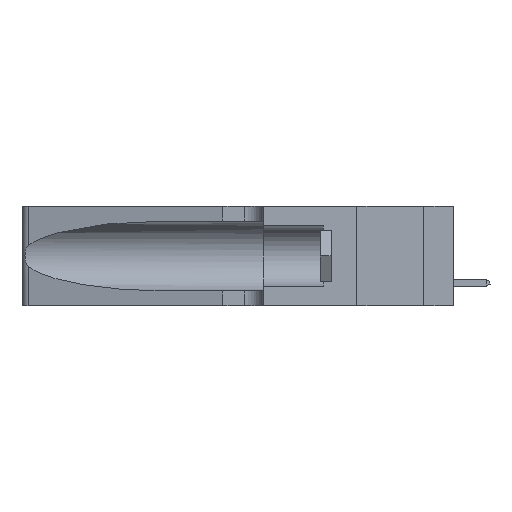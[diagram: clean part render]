
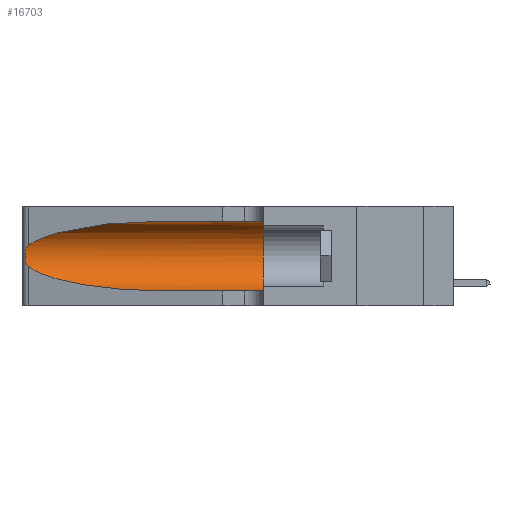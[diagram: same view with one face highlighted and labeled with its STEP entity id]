
A CAD part, left-side view. The second image highlights one B-rep face of the part: STEP entity #16703.
In plain terms, the highlighted cylindrical face has radius 3.308 mm (diameter 6.617 mm), a partial arc.
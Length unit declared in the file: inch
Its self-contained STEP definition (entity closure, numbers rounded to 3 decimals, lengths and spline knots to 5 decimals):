
#294 = VECTOR ( 'NONE', #23269, 39.37008 ) ;
#1287 = AXIS2_PLACEMENT_3D ( 'NONE', #34451, #16776, #19866 ) ;
#2170 = CARTESIAN_POINT ( 'NONE',  ( 0.26075, 1.23896, 0.178 ) ) ;
#2193 = CARTESIAN_POINT ( 'NONE',  ( 0.1305, 1.61858, 0.05475 ) ) ;
#3035 = CARTESIAN_POINT ( 'NONE',  ( 0.26017, 1.23833, 0.17102 ) ) ;
#4456 = CARTESIAN_POINT ( 'NONE',  ( 0.25487, 1.22718, 0.14631 ) ) ;
#4610 = VERTEX_POINT ( 'NONE', #22696 ) ;
#5009 = VERTEX_POINT ( 'NONE', #10681 ) ;
#5993 = ORIENTED_EDGE ( 'NONE', *, *, #29962, .T. ) ;
#7200 = DIRECTION ( 'NONE',  ( 0., 0., 1. ) ) ;
#7498 = CARTESIAN_POINT ( 'NONE',  ( 0.18966, 0.96281, 0.05475 ) ) ;
#8111 = CARTESIAN_POINT ( 'NONE',  ( 0.26075, 1.23896, 0.19203 ) ) ;
#8215 = VERTEX_POINT ( 'NONE', #34510 ) ;
#8740 = EDGE_LOOP ( 'NONE', ( #11631, #29557, #5993, #12788, #19186, #20772 ) ) ;
#9137 = EDGE_CURVE ( 'NONE', #5009, #36324, #16368, .T. ) ;
#9189 = AXIS2_PLACEMENT_3D ( 'NONE', #31284, #34332, #7200 ) ;
#9441 = CARTESIAN_POINT ( 'NONE',  ( 0.1305, 0.72297, 0.05475 ) ) ;
#10681 = CARTESIAN_POINT ( 'NONE',  ( 0.1305, 0.35, 0.31525 ) ) ;
#11172 = VECTOR ( 'NONE', #36040, 39.37008 ) ;
#11631 = ORIENTED_EDGE ( 'NONE', *, *, #24016, .T. ) ;
#11641 = LINE ( 'NONE', #29911, #11172 ) ;
#11677 = LINE ( 'NONE', #2193, #294 ) ;
#12788 = ORIENTED_EDGE ( 'NONE', *, *, #28646, .T. ) ;
#13900 = CARTESIAN_POINT ( 'NONE',  ( 0.25639, 1.23184, 0.21858 ) ) ;
#14667 = CARTESIAN_POINT ( 'NONE',  ( 0.25487, 1.22718, 0.14631 ) ) ;
#16368 = CIRCLE ( 'NONE', #9189, 0.13025 ) ;
#16436 =( BOUNDED_CURVE ( )  B_SPLINE_CURVE ( 3, ( #4456, #25472, #7498, #37796 ),
 .UNSPECIFIED., .F., .T. ) 
 B_SPLINE_CURVE_WITH_KNOTS ( ( 4, 4 ),
 ( 3.44316, 4.71239 ),
 .UNSPECIFIED. ) 
 CURVE ( )  GEOMETRIC_REPRESENTATION_ITEM ( )  RATIONAL_B_SPLINE_CURVE ( ( 1., 0.87, 0.87, 1. ) ) 
 REPRESENTATION_ITEM ( '' )  );
#16703 = ADVANCED_FACE ( 'NONE', ( #26738 ), #18725, .F. ) ;
#16776 = DIRECTION ( 'NONE',  ( 0., -1., 0. ) ) ;
#17062 = CARTESIAN_POINT ( 'NONE',  ( 0.26018, 1.23835, 0.19895 ) ) ;
#18725 = CYLINDRICAL_SURFACE ( 'NONE', #1287, 0.13025 ) ;
#19186 = ORIENTED_EDGE ( 'NONE', *, *, #9137, .F. ) ;
#19194 = EDGE_CURVE ( 'NONE', #8215, #21611, #33184, .T. ) ;
#19429 = CARTESIAN_POINT ( 'NONE',  ( 0.25555, 1.22994, 0.2215 ) ) ;
#19866 = DIRECTION ( 'NONE',  ( 0., 0., -1. ) ) ;
#20010 = CARTESIAN_POINT ( 'NONE',  ( 0.25787, 1.23484, 0.2124 ) ) ;
#20617 = CARTESIAN_POINT ( 'NONE',  ( 0.25639, 1.23186, 0.15144 ) ) ;
#20772 = ORIENTED_EDGE ( 'NONE', *, *, #29282, .F. ) ;
#21611 = VERTEX_POINT ( 'NONE', #29450 ) ;
#22696 = CARTESIAN_POINT ( 'NONE',  ( 0.1305, 0.72297, 0.31525 ) ) ;
#22858 = CARTESIAN_POINT ( 'NONE',  ( 0.25487, 1.22718, 0.22369 ) ) ;
#23269 = DIRECTION ( 'NONE',  ( 0., -1., 0. ) ) ;
#24016 = EDGE_CURVE ( 'NONE', #4610, #8215, #27942, .T. ) ;
#25472 = CARTESIAN_POINT ( 'NONE',  ( 0.2373, 1.15595, 0.08982 ) ) ;
#26592 = CARTESIAN_POINT ( 'NONE',  ( 0.25555, 1.22993, 0.14849 ) ) ;
#26738 = FACE_OUTER_BOUND ( 'NONE', #8740, .T. ) ;
#27559 = VERTEX_POINT ( 'NONE', #9441 ) ;
#27912 = CARTESIAN_POINT ( 'NONE',  ( 0.18966, 0.96281, 0.31525 ) ) ;
#27942 =( BOUNDED_CURVE ( )  B_SPLINE_CURVE ( 3, ( #28336, #27912, #31033, #30891 ),
 .UNSPECIFIED., .F., .T. ) 
 B_SPLINE_CURVE_WITH_KNOTS ( ( 4, 4 ),
 ( 1.5708, 2.84003 ),
 .UNSPECIFIED. ) 
 CURVE ( )  GEOMETRIC_REPRESENTATION_ITEM ( )  RATIONAL_B_SPLINE_CURVE ( ( 1., 0.87, 0.87, 1. ) ) 
 REPRESENTATION_ITEM ( '' )  );
#28336 = CARTESIAN_POINT ( 'NONE',  ( 0.1305, 0.72297, 0.31525 ) ) ;
#28646 = EDGE_CURVE ( 'NONE', #27559, #36324, #11677, .T. ) ;
#29282 = EDGE_CURVE ( 'NONE', #4610, #5009, #11641, .T. ) ;
#29450 = CARTESIAN_POINT ( 'NONE',  ( 0.25487, 1.22718, 0.14631 ) ) ;
#29495 = CARTESIAN_POINT ( 'NONE',  ( 0.25856, 1.23593, 0.16098 ) ) ;
#29557 = ORIENTED_EDGE ( 'NONE', *, *, #19194, .T. ) ;
#29911 = CARTESIAN_POINT ( 'NONE',  ( 0.1305, 1.61858, 0.31525 ) ) ;
#29962 = EDGE_CURVE ( 'NONE', #21611, #27559, #16436, .T. ) ;
#30891 = CARTESIAN_POINT ( 'NONE',  ( 0.25487, 1.22718, 0.22369 ) ) ;
#31033 = CARTESIAN_POINT ( 'NONE',  ( 0.2373, 1.15595, 0.28018 ) ) ;
#31284 = CARTESIAN_POINT ( 'NONE',  ( 0.1305, 0.35, 0.185 ) ) ;
#31930 = CARTESIAN_POINT ( 'NONE',  ( 0.25854, 1.2359, 0.20912 ) ) ;
#33184 = B_SPLINE_CURVE_WITH_KNOTS ( 'NONE', 3,
 ( #22858, #19429, #13900, #20010, #31930, #17062, #8111, #2170, #3035, #29495, #35489, #20617, #26592, #14667 ),
 .UNSPECIFIED., .F., .F.,
 ( 4, 2, 2, 2, 2, 2, 4 ),
 ( 0., 0.00027, 0.00053, 0.00107, 0.0016, 0.00187, 0.00214 ),
 .UNSPECIFIED. ) ;
#34332 = DIRECTION ( 'NONE',  ( 0., 1., 0. ) ) ;
#34451 = CARTESIAN_POINT ( 'NONE',  ( 0.1305, 1.61858, 0.185 ) ) ;
#34510 = CARTESIAN_POINT ( 'NONE',  ( 0.25487, 1.22718, 0.22369 ) ) ;
#35489 = CARTESIAN_POINT ( 'NONE',  ( 0.25789, 1.23486, 0.15765 ) ) ;
#35509 = CARTESIAN_POINT ( 'NONE',  ( 0.1305, 0.35, 0.05475 ) ) ;
#36040 = DIRECTION ( 'NONE',  ( 0., -1., 0. ) ) ;
#36324 = VERTEX_POINT ( 'NONE', #35509 ) ;
#37796 = CARTESIAN_POINT ( 'NONE',  ( 0.1305, 0.72297, 0.05475 ) ) ;
